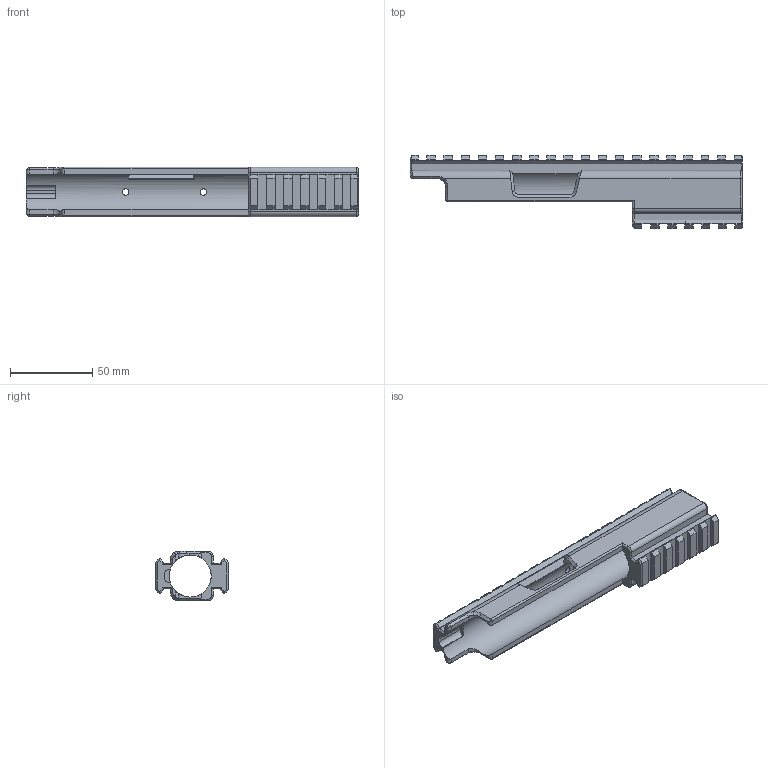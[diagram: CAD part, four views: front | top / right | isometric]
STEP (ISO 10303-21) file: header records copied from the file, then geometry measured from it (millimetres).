
FILE_DESCRIPTION(/* description */ (''),/* implementation_level */ '2;1');
FILE_NAME(/* name */ '2245 Lite Sleeve.step',/* time_stamp */ '2021-07-06T09:29:53-06:00',/* author */ (''),/* organization */ (''),/* preprocessor_version */ 'ST-DEVELOPER v18.1',/* originating_system */ 'Autodesk Translation Framework v10.9.0.1377',/* authorisation */ '');
FILE_SCHEMA (('AUTOMOTIVE_DESIGN { 1 0 10303 214 3 1 1 }'));
Length unit declared in the file: millimetre
Products named in the file (1): MK3
Bounding box: 201.5 x 44.32 x 30 mm (x, y, z)
Volume: 65906 mm3; surface area: 37168.5 mm2
Topology: 1 solids, 1 shells, 390 faces, 1000 edges, 607 vertices
Faces by surface type: plane 332, cylinder 36, bspline 10, torus 6, cone 6
Full cylindrical faces by diameter (mm): 4 x3, 6.5 x3, 25.5 x1
Entity records: 11880 total; most frequent: CARTESIAN_POINT 2513, ORIENTED_EDGE 2000, DIRECTION 1811, EDGE_CURVE 1000, LINE 873, VECTOR 873, VERTEX_POINT 607, AXIS2_PLACEMENT_3D 469
